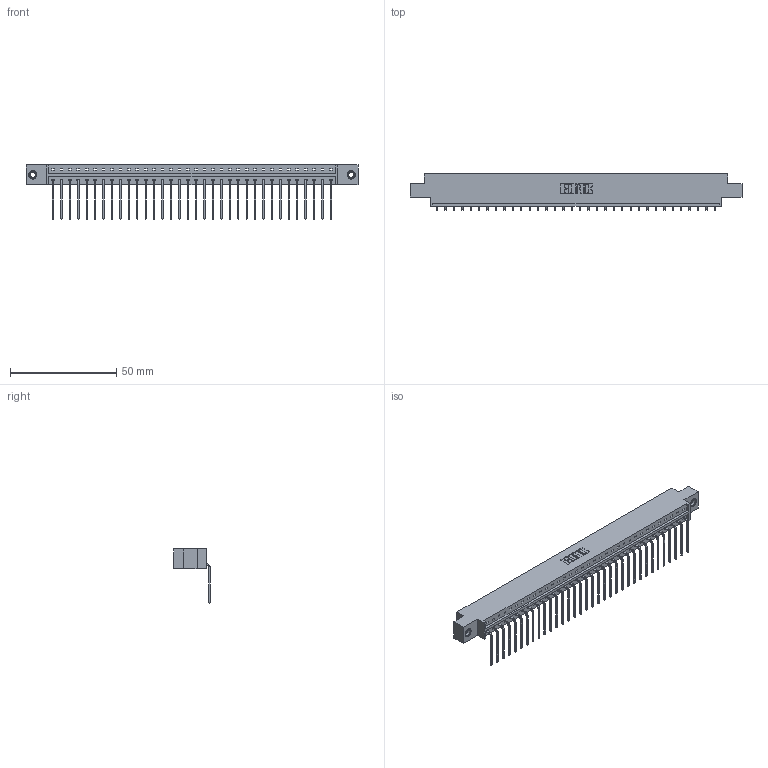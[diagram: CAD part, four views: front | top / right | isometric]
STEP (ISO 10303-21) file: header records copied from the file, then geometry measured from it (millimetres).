
FILE_DESCRIPTION (( 'STEP AP203' ), '1' );
FILE_NAME ('333-034-559-607.STEP', '2018-08-02T23:06:43', ( '' ), ( '' ), 'SwSTEP 2.0', 'SolidWorks 2016', '' );
FILE_SCHEMA (( 'CONFIG_CONTROL_DESIGN' ));
Length unit declared in the file: inch
Products named in the file (4): 345-292-001_558 559 Tail - 1; 345-250-001_345-250-005-103; 333-034-559-607; 333 Part_Offset - .156 Dia - TI
Assembly tree (37 placements, depth 2):
  333-034-559-607
    333 Part_Offset - .156 Dia - TI
    345-292-001_558 559 Tail - 1  x34
    345-250-001_345-250-005-103  x2
Bounding box: 156.26 x 17.09 x 25.53 mm (x, y, z)
Volume: 15527.4 mm3; surface area: 17678.2 mm2
Topology: 37 solids, 37 shells, 2218 faces, 6647 edges, 4378 vertices
Faces by surface type: plane 1602, cylinder 600, cone 12, torus 4
Entity records: 23222 total; most frequent: CARTESIAN_POINT 3991, ORIENTED_EDGE 3954, DIRECTION 3415, EDGE_CURVE 1977, VECTOR 1829, LINE 1829, VERTEX_POINT 1312, AXIS2_PLACEMENT_3D 793
